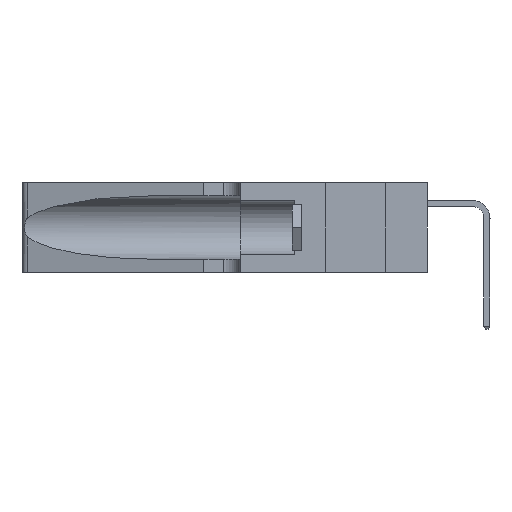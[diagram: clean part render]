
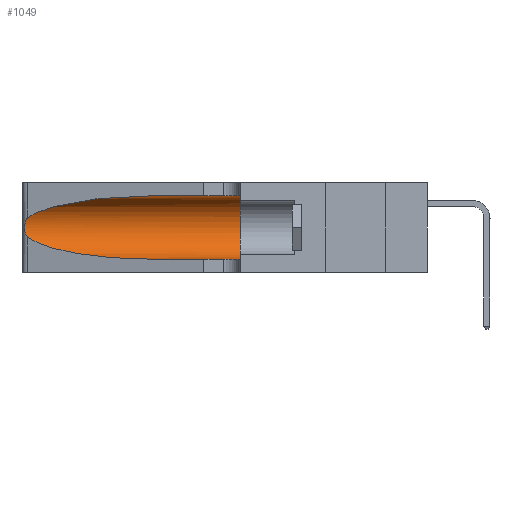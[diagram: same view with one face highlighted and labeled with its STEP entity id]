
A CAD part, left-side view. The second image highlights one B-rep face of the part: STEP entity #1049.
In plain terms, the highlighted cylindrical face has radius 3.308 mm (diameter 6.617 mm), a partial arc.
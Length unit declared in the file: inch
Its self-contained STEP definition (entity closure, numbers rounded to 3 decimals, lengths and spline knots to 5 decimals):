
#898 = DIRECTION ( 'NONE',  ( 0., 1., 0. ) ) ;
#1049 = ADVANCED_FACE ( 'NONE', ( #18399 ), #17617, .F. ) ;
#1130 = EDGE_CURVE ( 'NONE', #12594, #23358, #24499, .T. ) ;
#1444 = CARTESIAN_POINT ( 'NONE',  ( 0.25854, 1.2359, 0.20912 ) ) ;
#1520 = VERTEX_POINT ( 'NONE', #27071 ) ;
#3476 = EDGE_CURVE ( 'NONE', #8865, #4614, #26922, .T. ) ;
#3997 = CARTESIAN_POINT ( 'NONE',  ( 0.26075, 1.23896, 0.19203 ) ) ;
#4614 = VERTEX_POINT ( 'NONE', #21943 ) ;
#5598 = LINE ( 'NONE', #23588, #18253 ) ;
#5805 = ORIENTED_EDGE ( 'NONE', *, *, #13188, .T. ) ;
#6541 = CARTESIAN_POINT ( 'NONE',  ( 0.26017, 1.23833, 0.17102 ) ) ;
#6989 = ORIENTED_EDGE ( 'NONE', *, *, #3476, .T. ) ;
#7579 = EDGE_CURVE ( 'NONE', #1520, #32320, #32254, .T. ) ;
#7748 = CARTESIAN_POINT ( 'NONE',  ( 0.18966, 0.96281, 0.31525 ) ) ;
#8865 = VERTEX_POINT ( 'NONE', #21534 ) ;
#9075 = CARTESIAN_POINT ( 'NONE',  ( 0.25789, 1.23486, 0.15765 ) ) ;
#9489 = CARTESIAN_POINT ( 'NONE',  ( 0.1305, 0.72297, 0.05475 ) ) ;
#10040 = DIRECTION ( 'NONE',  ( 0., -1., 0. ) ) ;
#10087 = CARTESIAN_POINT ( 'NONE',  ( 0.1305, 1.61858, 0.185 ) ) ;
#11503 = AXIS2_PLACEMENT_3D ( 'NONE', #16093, #898, #18611 ) ;
#11646 = CARTESIAN_POINT ( 'NONE',  ( 0.25555, 1.22993, 0.14849 ) ) ;
#12137 = ORIENTED_EDGE ( 'NONE', *, *, #27791, .T. ) ;
#12594 = VERTEX_POINT ( 'NONE', #15470 ) ;
#12624 = DIRECTION ( 'NONE',  ( 0., 0., -1. ) ) ;
#12848 = CARTESIAN_POINT ( 'NONE',  ( 0.1305, 0.72297, 0.31525 ) ) ;
#13188 = EDGE_CURVE ( 'NONE', #4614, #32320, #5598, .T. ) ;
#15118 = CARTESIAN_POINT ( 'NONE',  ( 0.1305, 0.35, 0.05475 ) ) ;
#15400 = CARTESIAN_POINT ( 'NONE',  ( 0.25487, 1.22718, 0.22369 ) ) ;
#15470 = CARTESIAN_POINT ( 'NONE',  ( 0.1305, 0.72297, 0.31525 ) ) ;
#16093 = CARTESIAN_POINT ( 'NONE',  ( 0.1305, 0.35, 0.185 ) ) ;
#16407 = CARTESIAN_POINT ( 'NONE',  ( 0.25487, 1.22718, 0.22369 ) ) ;
#16620 = CARTESIAN_POINT ( 'NONE',  ( 0.25787, 1.23484, 0.2124 ) ) ;
#17617 = CYLINDRICAL_SURFACE ( 'NONE', #22435, 0.13025 ) ;
#18053 = ORIENTED_EDGE ( 'NONE', *, *, #1130, .T. ) ;
#18253 = VECTOR ( 'NONE', #26120, 39.37008 ) ;
#18399 = FACE_OUTER_BOUND ( 'NONE', #25684, .T. ) ;
#18611 = DIRECTION ( 'NONE',  ( 0., 0., 1. ) ) ;
#18871 = ORIENTED_EDGE ( 'NONE', *, *, #19301, .F. ) ;
#19152 = CARTESIAN_POINT ( 'NONE',  ( 0.26018, 1.23835, 0.19895 ) ) ;
#19301 = EDGE_CURVE ( 'NONE', #12594, #1520, #21141, .T. ) ;
#20363 = VECTOR ( 'NONE', #10040, 39.37008 ) ;
#21141 = LINE ( 'NONE', #25176, #20363 ) ;
#21534 = CARTESIAN_POINT ( 'NONE',  ( 0.25487, 1.22718, 0.14631 ) ) ;
#21692 = CARTESIAN_POINT ( 'NONE',  ( 0.26075, 1.23896, 0.178 ) ) ;
#21943 = CARTESIAN_POINT ( 'NONE',  ( 0.1305, 0.72297, 0.05475 ) ) ;
#22435 = AXIS2_PLACEMENT_3D ( 'NONE', #10087, #27743, #12624 ) ;
#23086 = B_SPLINE_CURVE_WITH_KNOTS ( 'NONE', 3,
 ( #16407, #24128, #31717, #16620, #1444, #19152, #3997, #21692, #6541, #24235, #9075, #26769, #11646, #29295 ),
 .UNSPECIFIED., .F., .F.,
 ( 4, 2, 2, 2, 2, 2, 4 ),
 ( 0., 0.00027, 0.00053, 0.00107, 0.0016, 0.00187, 0.00214 ),
 .UNSPECIFIED. ) ;
#23358 = VERTEX_POINT ( 'NONE', #31522 ) ;
#23588 = CARTESIAN_POINT ( 'NONE',  ( 0.1305, 1.61858, 0.05475 ) ) ;
#24128 = CARTESIAN_POINT ( 'NONE',  ( 0.25555, 1.22994, 0.2215 ) ) ;
#24235 = CARTESIAN_POINT ( 'NONE',  ( 0.25856, 1.23593, 0.16098 ) ) ;
#24499 =( BOUNDED_CURVE ( )  B_SPLINE_CURVE ( 3, ( #12848, #7748, #30370, #15400 ),
 .UNSPECIFIED., .F., .F. ) 
 B_SPLINE_CURVE_WITH_KNOTS ( ( 4, 4 ),
 ( 1.5708, 2.84003 ),
 .UNSPECIFIED. ) 
 CURVE ( )  GEOMETRIC_REPRESENTATION_ITEM ( )  RATIONAL_B_SPLINE_CURVE ( ( 1., 0.87, 0.87, 1. ) ) 
 REPRESENTATION_ITEM ( '' )  );
#24650 = CARTESIAN_POINT ( 'NONE',  ( 0.25487, 1.22718, 0.14631 ) ) ;
#25176 = CARTESIAN_POINT ( 'NONE',  ( 0.1305, 1.61858, 0.31525 ) ) ;
#25684 = EDGE_LOOP ( 'NONE', ( #18053, #12137, #6989, #5805, #26766, #18871 ) ) ;
#26120 = DIRECTION ( 'NONE',  ( 0., -1., 0. ) ) ;
#26766 = ORIENTED_EDGE ( 'NONE', *, *, #7579, .F. ) ;
#26769 = CARTESIAN_POINT ( 'NONE',  ( 0.25639, 1.23186, 0.15144 ) ) ;
#26922 =( BOUNDED_CURVE ( )  B_SPLINE_CURVE ( 3, ( #24650, #26958, #29588, #9489 ),
 .UNSPECIFIED., .F., .F. ) 
 B_SPLINE_CURVE_WITH_KNOTS ( ( 4, 4 ),
 ( 3.44316, 4.71239 ),
 .UNSPECIFIED. ) 
 CURVE ( )  GEOMETRIC_REPRESENTATION_ITEM ( )  RATIONAL_B_SPLINE_CURVE ( ( 1., 0.87, 0.87, 1. ) ) 
 REPRESENTATION_ITEM ( '' )  );
#26958 = CARTESIAN_POINT ( 'NONE',  ( 0.2373, 1.15595, 0.08982 ) ) ;
#27071 = CARTESIAN_POINT ( 'NONE',  ( 0.1305, 0.35, 0.31525 ) ) ;
#27743 = DIRECTION ( 'NONE',  ( 0., -1., 0. ) ) ;
#27791 = EDGE_CURVE ( 'NONE', #23358, #8865, #23086, .T. ) ;
#29295 = CARTESIAN_POINT ( 'NONE',  ( 0.25487, 1.22718, 0.14631 ) ) ;
#29588 = CARTESIAN_POINT ( 'NONE',  ( 0.18966, 0.96281, 0.05475 ) ) ;
#30370 = CARTESIAN_POINT ( 'NONE',  ( 0.2373, 1.15595, 0.28018 ) ) ;
#31522 = CARTESIAN_POINT ( 'NONE',  ( 0.25487, 1.22718, 0.22369 ) ) ;
#31717 = CARTESIAN_POINT ( 'NONE',  ( 0.25639, 1.23184, 0.21858 ) ) ;
#32254 = CIRCLE ( 'NONE', #11503, 0.13025 ) ;
#32320 = VERTEX_POINT ( 'NONE', #15118 ) ;
